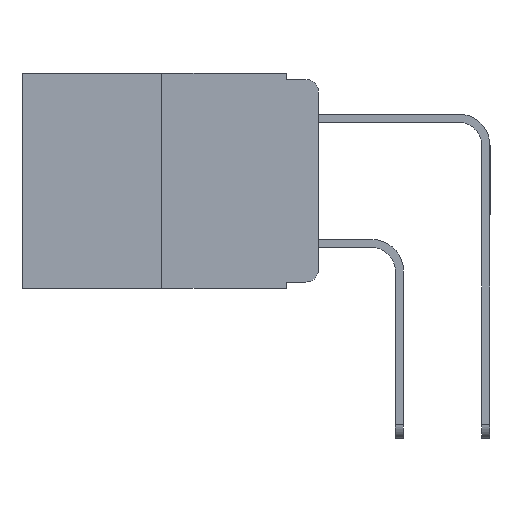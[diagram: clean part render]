
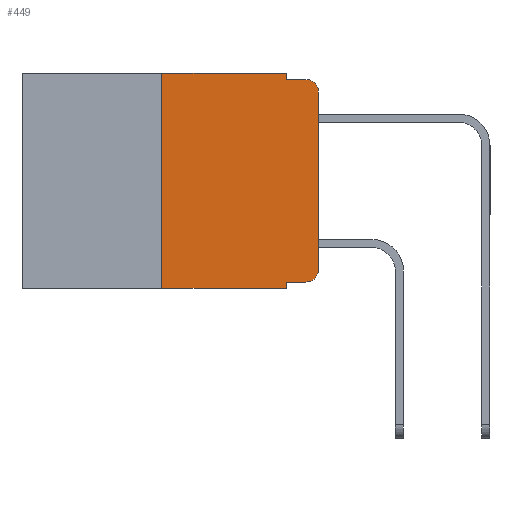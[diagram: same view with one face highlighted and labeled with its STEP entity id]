
A CAD part, left-side view. The second image highlights one B-rep face of the part: STEP entity #449.
In plain terms, the highlighted planar face has unit normal (-1, 0, 0).
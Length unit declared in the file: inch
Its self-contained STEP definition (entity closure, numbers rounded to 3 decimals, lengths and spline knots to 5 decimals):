
#259 = CARTESIAN_POINT ( 'NONE',  ( 0., 0.051, 0. ) ) ;
#376 = EDGE_LOOP ( 'NONE', ( #10614, #14078, #17575, #1506, #9000, #6018, #14222, #852, #2783, #14591 ) ) ;
#387 = VERTEX_POINT ( 'NONE', #14236 ) ;
#424 = LINE ( 'NONE', #16987, #18097 ) ;
#449 = ADVANCED_FACE ( 'NONE', ( #20092 ), #12450, .F. ) ;
#832 = DIRECTION ( 'NONE',  ( 0., 0., -1. ) ) ;
#851 = CARTESIAN_POINT ( 'NONE',  ( 0., 0., 0. ) ) ;
#852 = ORIENTED_EDGE ( 'NONE', *, *, #5838, .F. ) ;
#1307 = VECTOR ( 'NONE', #14728, 39.37008 ) ;
#1439 = CIRCLE ( 'NONE', #4613, 0.02 ) ;
#1506 = ORIENTED_EDGE ( 'NONE', *, *, #8265, .F. ) ;
#1749 = CARTESIAN_POINT ( 'NONE',  ( 0., 0.25, -0.343 ) ) ;
#2180 = LINE ( 'NONE', #13063, #11054 ) ;
#2189 = EDGE_CURVE ( 'NONE', #19641, #5952, #4241, .T. ) ;
#2450 = VERTEX_POINT ( 'NONE', #11794 ) ;
#2599 = CARTESIAN_POINT ( 'NONE',  ( 0., 0.25, 0. ) ) ;
#2660 = DIRECTION ( 'NONE',  ( 0., 0., 1. ) ) ;
#2689 = VERTEX_POINT ( 'NONE', #1749 ) ;
#2783 = ORIENTED_EDGE ( 'NONE', *, *, #3402, .T. ) ;
#3402 = EDGE_CURVE ( 'NONE', #2450, #19641, #2180, .T. ) ;
#4064 = VERTEX_POINT ( 'NONE', #5104 ) ;
#4241 = CIRCLE ( 'NONE', #11221, 0.02 ) ;
#4426 = DIRECTION ( 'NONE',  ( 0., 0., -1. ) ) ;
#4613 = AXIS2_PLACEMENT_3D ( 'NONE', #8489, #19975, #10161 ) ;
#4804 = DIRECTION ( 'NONE',  ( 0., 0., -1. ) ) ;
#5001 = LINE ( 'NONE', #851, #13568 ) ;
#5104 = CARTESIAN_POINT ( 'NONE',  ( 0., 0.051, -0.343 ) ) ;
#5187 = CARTESIAN_POINT ( 'NONE',  ( 0., 0., -0.313 ) ) ;
#5561 = CARTESIAN_POINT ( 'NONE',  ( 0., 0.02, -0.01 ) ) ;
#5676 = DIRECTION ( 'NONE',  ( -1., 0., 0. ) ) ;
#5838 = EDGE_CURVE ( 'NONE', #2450, #4064, #8753, .T. ) ;
#5952 = VERTEX_POINT ( 'NONE', #5187 ) ;
#6018 = ORIENTED_EDGE ( 'NONE', *, *, #7065, .F. ) ;
#7065 = EDGE_CURVE ( 'NONE', #2689, #22045, #17375, .T. ) ;
#8265 = EDGE_CURVE ( 'NONE', #11968, #18751, #20174, .T. ) ;
#8347 = DIRECTION ( 'NONE',  ( 0., 0., -1. ) ) ;
#8379 = DIRECTION ( 'NONE',  ( 1., 0., 0. ) ) ;
#8489 = CARTESIAN_POINT ( 'NONE',  ( 0., 0.02, -0.03 ) ) ;
#8502 = DIRECTION ( 'NONE',  ( 0., 0., 1. ) ) ;
#8753 = LINE ( 'NONE', #18229, #16935 ) ;
#9000 = ORIENTED_EDGE ( 'NONE', *, *, #15879, .F. ) ;
#9428 = EDGE_CURVE ( 'NONE', #18751, #17485, #424, .T. ) ;
#9754 = CARTESIAN_POINT ( 'NONE',  ( 0., 0.473, 0. ) ) ;
#10161 = DIRECTION ( 'NONE',  ( 0., 0., -1. ) ) ;
#10239 = LINE ( 'NONE', #19758, #14121 ) ;
#10614 = ORIENTED_EDGE ( 'NONE', *, *, #12786, .T. ) ;
#11054 = VECTOR ( 'NONE', #14303, 39.37008 ) ;
#11192 = CARTESIAN_POINT ( 'NONE',  ( 0., 0.02, -0.333 ) ) ;
#11221 = AXIS2_PLACEMENT_3D ( 'NONE', #13513, #5676, #832 ) ;
#11515 = VECTOR ( 'NONE', #4426, 39.37008 ) ;
#11655 = EDGE_CURVE ( 'NONE', #387, #17485, #1439, .T. ) ;
#11794 = CARTESIAN_POINT ( 'NONE',  ( 0., 0.051, -0.333 ) ) ;
#11863 = CARTESIAN_POINT ( 'NONE',  ( 0., 0.25, 0. ) ) ;
#11968 = VERTEX_POINT ( 'NONE', #259 ) ;
#12450 = PLANE ( 'NONE',  #15695 ) ;
#12786 = EDGE_CURVE ( 'NONE', #5952, #387, #5001, .T. ) ;
#13063 = CARTESIAN_POINT ( 'NONE',  ( 0., 0.051, -0.333 ) ) ;
#13513 = CARTESIAN_POINT ( 'NONE',  ( 0., 0.02, -0.313 ) ) ;
#13568 = VECTOR ( 'NONE', #2660, 39.37008 ) ;
#14078 = ORIENTED_EDGE ( 'NONE', *, *, #11655, .T. ) ;
#14121 = VECTOR ( 'NONE', #18089, 39.37008 ) ;
#14222 = ORIENTED_EDGE ( 'NONE', *, *, #16660, .T. ) ;
#14236 = CARTESIAN_POINT ( 'NONE',  ( 0., 0., -0.03 ) ) ;
#14303 = DIRECTION ( 'NONE',  ( 0., -1., 0. ) ) ;
#14591 = ORIENTED_EDGE ( 'NONE', *, *, #2189, .T. ) ;
#14728 = DIRECTION ( 'NONE',  ( 0., -1., 0. ) ) ;
#15695 = AXIS2_PLACEMENT_3D ( 'NONE', #21822, #8379, #8347 ) ;
#15879 = EDGE_CURVE ( 'NONE', #22045, #11968, #19461, .T. ) ;
#16248 = CARTESIAN_POINT ( 'NONE',  ( 0., 0.051, 0. ) ) ;
#16660 = EDGE_CURVE ( 'NONE', #2689, #4064, #10239, .T. ) ;
#16935 = VECTOR ( 'NONE', #4804, 39.37008 ) ;
#16987 = CARTESIAN_POINT ( 'NONE',  ( 0., 0.051, -0.01 ) ) ;
#17095 = CARTESIAN_POINT ( 'NONE',  ( 0., 0.051, -0.01 ) ) ;
#17375 = LINE ( 'NONE', #11863, #21760 ) ;
#17485 = VERTEX_POINT ( 'NONE', #5561 ) ;
#17575 = ORIENTED_EDGE ( 'NONE', *, *, #9428, .F. ) ;
#18089 = DIRECTION ( 'NONE',  ( 0., -1., 0. ) ) ;
#18097 = VECTOR ( 'NONE', #18653, 39.37008 ) ;
#18229 = CARTESIAN_POINT ( 'NONE',  ( 0., 0.051, 0. ) ) ;
#18653 = DIRECTION ( 'NONE',  ( 0., -1., 0. ) ) ;
#18751 = VERTEX_POINT ( 'NONE', #17095 ) ;
#19461 = LINE ( 'NONE', #9754, #1307 ) ;
#19641 = VERTEX_POINT ( 'NONE', #11192 ) ;
#19758 = CARTESIAN_POINT ( 'NONE',  ( 0., 0.473, -0.343 ) ) ;
#19975 = DIRECTION ( 'NONE',  ( -1., 0., 0. ) ) ;
#20092 = FACE_OUTER_BOUND ( 'NONE', #376, .T. ) ;
#20174 = LINE ( 'NONE', #16248, #11515 ) ;
#21760 = VECTOR ( 'NONE', #8502, 39.37008 ) ;
#21822 = CARTESIAN_POINT ( 'NONE',  ( 0., 0.473, 0. ) ) ;
#22045 = VERTEX_POINT ( 'NONE', #2599 ) ;
